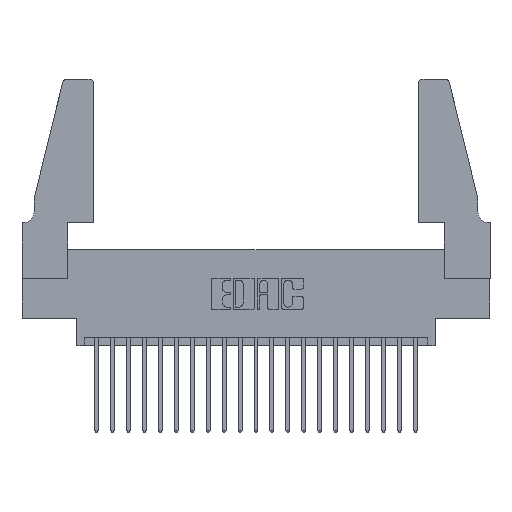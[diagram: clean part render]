
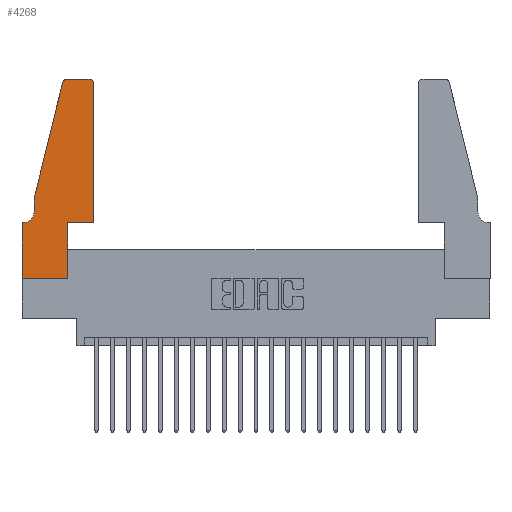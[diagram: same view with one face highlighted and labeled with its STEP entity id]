
A CAD part, top view. The second image highlights one B-rep face of the part: STEP entity #4268.
In plain terms, the highlighted planar face has unit normal (0, 0, 1).
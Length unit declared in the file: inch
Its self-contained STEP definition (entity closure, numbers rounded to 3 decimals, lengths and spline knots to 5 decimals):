
#86 = VECTOR ( 'NONE', #18677, 39.37008 ) ;
#351 = CARTESIAN_POINT ( 'NONE',  ( 0.4505, 0.35, 0.37 ) ) ;
#451 = DIRECTION ( 'NONE',  ( 1., 0., 0. ) ) ;
#757 = AXIS2_PLACEMENT_3D ( 'NONE', #13824, #2073, #20322 ) ;
#967 = CARTESIAN_POINT ( 'NONE',  ( 0.0055, 0.42, 0.37 ) ) ;
#1173 = CARTESIAN_POINT ( 'NONE',  ( 0.0755, 0.5, 0.37 ) ) ;
#1554 = ORIENTED_EDGE ( 'NONE', *, *, #13218, .T. ) ;
#2068 = LINE ( 'NONE', #1173, #14903 ) ;
#2073 = DIRECTION ( 'NONE',  ( 0., 0., 1. ) ) ;
#2266 = VECTOR ( 'NONE', #5509, 39.37008 ) ;
#2654 = CARTESIAN_POINT ( 'NONE',  ( 0.4205, 1.25, 0.37 ) ) ;
#2744 = DIRECTION ( 'NONE',  ( -1., 0., 0. ) ) ;
#2876 = CARTESIAN_POINT ( 'NONE',  ( 0., 0., 0.37 ) ) ;
#2940 = LINE ( 'NONE', #4093, #11381 ) ;
#3330 = VECTOR ( 'NONE', #451, 39.37008 ) ;
#3788 = CARTESIAN_POINT ( 'NONE',  ( 0.0755, 0.5, 0.37 ) ) ;
#4093 = CARTESIAN_POINT ( 'NONE',  ( 0.4505, 0.35, 0.37 ) ) ;
#4155 = VERTEX_POINT ( 'NONE', #5259 ) ;
#4255 = ORIENTED_EDGE ( 'NONE', *, *, #12773, .T. ) ;
#4268 = ADVANCED_FACE ( 'NONE', ( #21435 ), #17106, .T. ) ;
#4690 = CIRCLE ( 'NONE', #19808, 0.03 ) ;
#4755 = CARTESIAN_POINT ( 'NONE',  ( 0.2865, 0.35, 0.37 ) ) ;
#4803 = VECTOR ( 'NONE', #20435, 39.37008 ) ;
#4881 = ORIENTED_EDGE ( 'NONE', *, *, #8347, .T. ) ;
#5035 = CARTESIAN_POINT ( 'NONE',  ( 0.284, 1.25, 0.37 ) ) ;
#5259 = CARTESIAN_POINT ( 'NONE',  ( 0.0755, 0.5, 0.37 ) ) ;
#5509 = DIRECTION ( 'NONE',  ( 0., -1., 0. ) ) ;
#5511 = CARTESIAN_POINT ( 'NONE',  ( 0.0755, 0.35, 0.37 ) ) ;
#5803 = DIRECTION ( 'NONE',  ( 0., 1., 0. ) ) ;
#6635 = VERTEX_POINT ( 'NONE', #17564 ) ;
#6950 = VECTOR ( 'NONE', #20951, 39.37008 ) ;
#7129 = ORIENTED_EDGE ( 'NONE', *, *, #9872, .T. ) ;
#7494 = VECTOR ( 'NONE', #17232, 39.37008 ) ;
#8280 = VERTEX_POINT ( 'NONE', #20069 ) ;
#8318 = CARTESIAN_POINT ( 'NONE',  ( 0., 0.35, 0.37 ) ) ;
#8347 = EDGE_CURVE ( 'NONE', #11279, #14813, #17992, .T. ) ;
#8410 = EDGE_LOOP ( 'NONE', ( #1554, #7129, #13208, #15817, #16278, #4881, #10065, #19888, #9815, #10815, #9570, #4255 ) ) ;
#8888 = LINE ( 'NONE', #17233, #3330 ) ;
#9057 = CARTESIAN_POINT ( 'NONE',  ( 0.2865, 0.35, 0.37 ) ) ;
#9478 = CARTESIAN_POINT ( 'NONE',  ( 0.0755, 0.42, 0.37 ) ) ;
#9502 = VERTEX_POINT ( 'NONE', #5035 ) ;
#9570 = ORIENTED_EDGE ( 'NONE', *, *, #17088, .T. ) ;
#9644 = DIRECTION ( 'NONE',  ( 0., 0., 1. ) ) ;
#9690 = EDGE_CURVE ( 'NONE', #20077, #12636, #8888, .T. ) ;
#9815 = ORIENTED_EDGE ( 'NONE', *, *, #16396, .T. ) ;
#9872 = EDGE_CURVE ( 'NONE', #9502, #17468, #4690, .T. ) ;
#9881 = DIRECTION ( 'NONE',  ( 0., 0., 1. ) ) ;
#10065 = ORIENTED_EDGE ( 'NONE', *, *, #13868, .T. ) ;
#10815 = ORIENTED_EDGE ( 'NONE', *, *, #17972, .T. ) ;
#11183 = CARTESIAN_POINT ( 'NONE',  ( 0.2865, 0., 0.37 ) ) ;
#11279 = VERTEX_POINT ( 'NONE', #14606 ) ;
#11372 = CIRCLE ( 'NONE', #14036, 0.03 ) ;
#11381 = VECTOR ( 'NONE', #5803, 39.37008 ) ;
#11566 = VECTOR ( 'NONE', #12926, 39.37008 ) ;
#11775 = LINE ( 'NONE', #3788, #2266 ) ;
#12079 = LINE ( 'NONE', #2876, #11566 ) ;
#12636 = VERTEX_POINT ( 'NONE', #11183 ) ;
#12773 = EDGE_CURVE ( 'NONE', #8280, #16559, #11372, .T. ) ;
#12818 = DIRECTION ( 'NONE',  ( 0., 0., -1. ) ) ;
#12926 = DIRECTION ( 'NONE',  ( 0., -1., 0. ) ) ;
#13181 = EDGE_CURVE ( 'NONE', #17223, #11279, #16715, .T. ) ;
#13208 = ORIENTED_EDGE ( 'NONE', *, *, #18125, .T. ) ;
#13218 = EDGE_CURVE ( 'NONE', #16559, #9502, #15694, .T. ) ;
#13346 = CARTESIAN_POINT ( 'NONE',  ( 0.25487, 1.22718, 0.37 ) ) ;
#13628 = LINE ( 'NONE', #351, #4803 ) ;
#13824 = CARTESIAN_POINT ( 'NONE',  ( 0., 0.35, 0.37 ) ) ;
#13868 = EDGE_CURVE ( 'NONE', #14813, #20077, #12079, .T. ) ;
#14036 = AXIS2_PLACEMENT_3D ( 'NONE', #19610, #9881, #21243 ) ;
#14527 = CARTESIAN_POINT ( 'NONE',  ( 0.2605, 1.25, 0.37 ) ) ;
#14606 = CARTESIAN_POINT ( 'NONE',  ( 0.0055, 0.35, 0.37 ) ) ;
#14644 = DIRECTION ( 'NONE',  ( -0.239, -0.971, 0. ) ) ;
#14778 = CARTESIAN_POINT ( 'NONE',  ( 0., 0., 0.37 ) ) ;
#14813 = VERTEX_POINT ( 'NONE', #8318 ) ;
#14903 = VECTOR ( 'NONE', #14644, 39.37008 ) ;
#15019 = EDGE_CURVE ( 'NONE', #4155, #17223, #11775, .T. ) ;
#15694 = LINE ( 'NONE', #14527, #6950 ) ;
#15817 = ORIENTED_EDGE ( 'NONE', *, *, #15019, .T. ) ;
#16013 = VERTEX_POINT ( 'NONE', #4755 ) ;
#16278 = ORIENTED_EDGE ( 'NONE', *, *, #13181, .T. ) ;
#16396 = EDGE_CURVE ( 'NONE', #12636, #16013, #20503, .T. ) ;
#16559 = VERTEX_POINT ( 'NONE', #2654 ) ;
#16715 = CIRCLE ( 'NONE', #16892, 0.07 ) ;
#16892 = AXIS2_PLACEMENT_3D ( 'NONE', #967, #12818, #2744 ) ;
#17088 = EDGE_CURVE ( 'NONE', #6635, #8280, #2940, .T. ) ;
#17106 = PLANE ( 'NONE',  #757 ) ;
#17223 = VERTEX_POINT ( 'NONE', #9478 ) ;
#17232 = DIRECTION ( 'NONE',  ( 0., 1., 0. ) ) ;
#17233 = CARTESIAN_POINT ( 'NONE',  ( 0., 0., 0.37 ) ) ;
#17468 = VERTEX_POINT ( 'NONE', #13346 ) ;
#17564 = CARTESIAN_POINT ( 'NONE',  ( 0.4505, 0.35, 0.37 ) ) ;
#17972 = EDGE_CURVE ( 'NONE', #16013, #6635, #13628, .T. ) ;
#17992 = LINE ( 'NONE', #5511, #86 ) ;
#18125 = EDGE_CURVE ( 'NONE', #17468, #4155, #2068, .T. ) ;
#18677 = DIRECTION ( 'NONE',  ( -1., 0., 0. ) ) ;
#19392 = CARTESIAN_POINT ( 'NONE',  ( 0.284, 1.22, 0.37 ) ) ;
#19610 = CARTESIAN_POINT ( 'NONE',  ( 0.4205, 1.22, 0.37 ) ) ;
#19808 = AXIS2_PLACEMENT_3D ( 'NONE', #19392, #9644, #21006 ) ;
#19888 = ORIENTED_EDGE ( 'NONE', *, *, #9690, .T. ) ;
#20069 = CARTESIAN_POINT ( 'NONE',  ( 0.4505, 1.22, 0.37 ) ) ;
#20077 = VERTEX_POINT ( 'NONE', #14778 ) ;
#20322 = DIRECTION ( 'NONE',  ( 1., 0., 0. ) ) ;
#20435 = DIRECTION ( 'NONE',  ( 1., 0., 0. ) ) ;
#20503 = LINE ( 'NONE', #9057, #7494 ) ;
#20951 = DIRECTION ( 'NONE',  ( -1., 0., 0. ) ) ;
#21006 = DIRECTION ( 'NONE',  ( 1., 0., 0. ) ) ;
#21243 = DIRECTION ( 'NONE',  ( 1., 0., 0. ) ) ;
#21435 = FACE_OUTER_BOUND ( 'NONE', #8410, .T. ) ;
